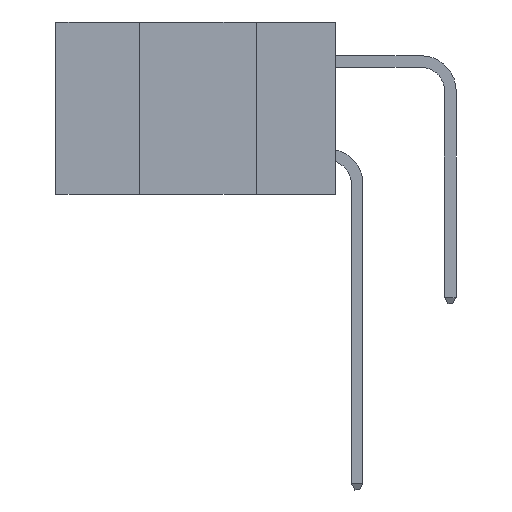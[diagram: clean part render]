
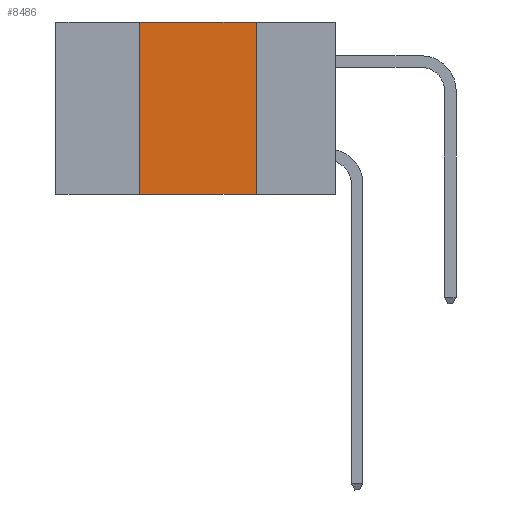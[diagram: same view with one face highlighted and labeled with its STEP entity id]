
A CAD part, left-side view. The second image highlights one B-rep face of the part: STEP entity #8486.
In plain terms, the highlighted planar face has unit normal (-1, 0, 0).
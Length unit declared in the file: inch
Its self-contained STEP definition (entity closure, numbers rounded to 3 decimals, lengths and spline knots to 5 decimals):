
#598 = CARTESIAN_POINT ( 'NONE',  ( 0., 0.17, 0. ) ) ;
#897 = LINE ( 'NONE', #12816, #14257 ) ;
#1685 = VERTEX_POINT ( 'NONE', #10492 ) ;
#1704 = CARTESIAN_POINT ( 'NONE',  ( 0., 0.17, 0. ) ) ;
#1777 = FACE_OUTER_BOUND ( 'NONE', #10391, .T. ) ;
#1957 = VERTEX_POINT ( 'NONE', #1704 ) ;
#2623 = CARTESIAN_POINT ( 'NONE',  ( 0., 0.42, -0.37 ) ) ;
#2688 = DIRECTION ( 'NONE',  ( 0., 0., -1. ) ) ;
#3122 = LINE ( 'NONE', #598, #13209 ) ;
#3836 = CARTESIAN_POINT ( 'NONE',  ( 0., 0.6, 0. ) ) ;
#3879 = LINE ( 'NONE', #4800, #6563 ) ;
#4409 = DIRECTION ( 'NONE',  ( 0., 0., -1. ) ) ;
#4799 = ORIENTED_EDGE ( 'NONE', *, *, #10410, .T. ) ;
#4800 = CARTESIAN_POINT ( 'NONE',  ( 0., 0.42, 0. ) ) ;
#5111 = VERTEX_POINT ( 'NONE', #2623 ) ;
#5325 = CARTESIAN_POINT ( 'NONE',  ( 0., 0.17, -0.37 ) ) ;
#5340 = EDGE_CURVE ( 'NONE', #5111, #1685, #3879, .T. ) ;
#5934 = EDGE_CURVE ( 'NONE', #1957, #7079, #3122, .T. ) ;
#5958 = DIRECTION ( 'NONE',  ( 0., 0., 1. ) ) ;
#6563 = VECTOR ( 'NONE', #5958, 39.37008 ) ;
#6773 = EDGE_CURVE ( 'NONE', #1685, #1957, #897, .T. ) ;
#6811 = VECTOR ( 'NONE', #11987, 39.37008 ) ;
#7079 = VERTEX_POINT ( 'NONE', #5325 ) ;
#8078 = LINE ( 'NONE', #14188, #6811 ) ;
#8486 = ADVANCED_FACE ( 'NONE', ( #1777 ), #9623, .F. ) ;
#9456 = ORIENTED_EDGE ( 'NONE', *, *, #5934, .F. ) ;
#9623 = PLANE ( 'NONE',  #12404 ) ;
#10391 = EDGE_LOOP ( 'NONE', ( #9456, #10859, #15028, #4799 ) ) ;
#10410 = EDGE_CURVE ( 'NONE', #5111, #7079, #8078, .T. ) ;
#10492 = CARTESIAN_POINT ( 'NONE',  ( 0., 0.42, 0. ) ) ;
#10859 = ORIENTED_EDGE ( 'NONE', *, *, #6773, .F. ) ;
#11337 = DIRECTION ( 'NONE',  ( 1., 0., 0. ) ) ;
#11987 = DIRECTION ( 'NONE',  ( 0., -1., 0. ) ) ;
#12404 = AXIS2_PLACEMENT_3D ( 'NONE', #3836, #11337, #4409 ) ;
#12816 = CARTESIAN_POINT ( 'NONE',  ( 0., 0.6, 0. ) ) ;
#13209 = VECTOR ( 'NONE', #2688, 39.37008 ) ;
#14188 = CARTESIAN_POINT ( 'NONE',  ( 0., 0.6, -0.37 ) ) ;
#14257 = VECTOR ( 'NONE', #15006, 39.37008 ) ;
#15006 = DIRECTION ( 'NONE',  ( 0., -1., 0. ) ) ;
#15028 = ORIENTED_EDGE ( 'NONE', *, *, #5340, .F. ) ;
